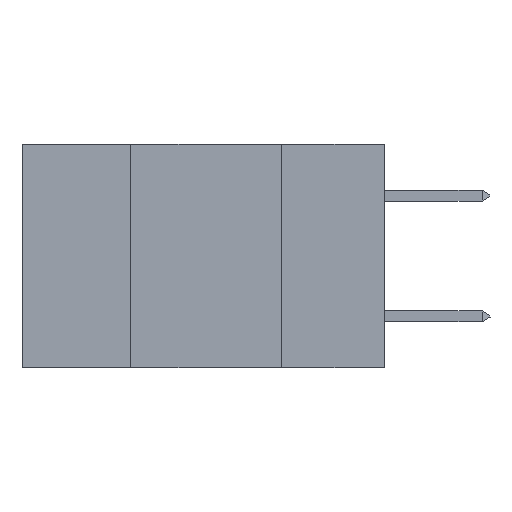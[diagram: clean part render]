
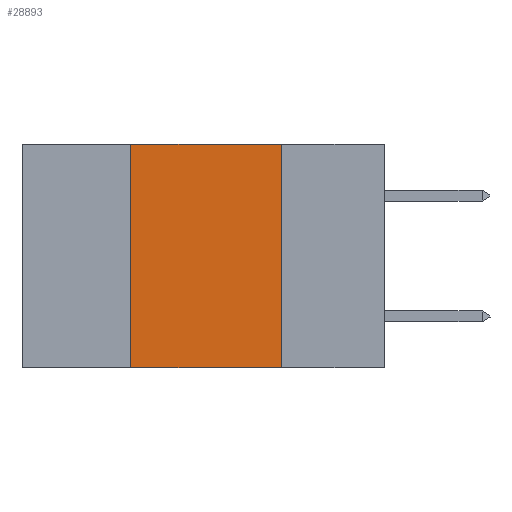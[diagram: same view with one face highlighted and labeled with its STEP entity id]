
A CAD part, left-side view. The second image highlights one B-rep face of the part: STEP entity #28893.
In plain terms, the highlighted planar face has unit normal (-1, 0, 0).
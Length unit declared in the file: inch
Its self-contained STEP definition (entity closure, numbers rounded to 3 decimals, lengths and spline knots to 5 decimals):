
#1052 = CARTESIAN_POINT ( 'NONE',  ( 0., 0.17, -0.37 ) ) ;
#1614 = ORIENTED_EDGE ( 'NONE', *, *, #23762, .F. ) ;
#2181 = FACE_OUTER_BOUND ( 'NONE', #28817, .T. ) ;
#2776 = EDGE_CURVE ( 'NONE', #21338, #18415, #12879, .T. ) ;
#3061 = LINE ( 'NONE', #16066, #25150 ) ;
#3311 = DIRECTION ( 'NONE',  ( 0., -1., 0. ) ) ;
#3324 = DIRECTION ( 'NONE',  ( 0., 0., 1. ) ) ;
#5458 = ORIENTED_EDGE ( 'NONE', *, *, #2776, .T. ) ;
#6096 = VECTOR ( 'NONE', #20080, 39.37008 ) ;
#8983 = CARTESIAN_POINT ( 'NONE',  ( 0., 0.42, -0.37 ) ) ;
#10614 = CARTESIAN_POINT ( 'NONE',  ( 0., 0.6, 0. ) ) ;
#11341 = VERTEX_POINT ( 'NONE', #28186 ) ;
#12218 = ORIENTED_EDGE ( 'NONE', *, *, #23630, .F. ) ;
#12879 = LINE ( 'NONE', #32663, #6096 ) ;
#14375 = CARTESIAN_POINT ( 'NONE',  ( 0., 0.17, 0. ) ) ;
#15922 = CARTESIAN_POINT ( 'NONE',  ( 0., 0.17, 0. ) ) ;
#16066 = CARTESIAN_POINT ( 'NONE',  ( 0., 0.42, 0. ) ) ;
#16925 = DIRECTION ( 'NONE',  ( 1., 0., 0. ) ) ;
#17274 = AXIS2_PLACEMENT_3D ( 'NONE', #32327, #16925, #19282 ) ;
#18415 = VERTEX_POINT ( 'NONE', #1052 ) ;
#19282 = DIRECTION ( 'NONE',  ( 0., 0., -1. ) ) ;
#20080 = DIRECTION ( 'NONE',  ( 0., -1., 0. ) ) ;
#20553 = VERTEX_POINT ( 'NONE', #14375 ) ;
#21338 = VERTEX_POINT ( 'NONE', #8983 ) ;
#21437 = VECTOR ( 'NONE', #28857, 39.37008 ) ;
#22272 = VECTOR ( 'NONE', #3311, 39.37008 ) ;
#22944 = EDGE_CURVE ( 'NONE', #21338, #11341, #3061, .T. ) ;
#23630 = EDGE_CURVE ( 'NONE', #20553, #18415, #27894, .T. ) ;
#23762 = EDGE_CURVE ( 'NONE', #11341, #20553, #25463, .T. ) ;
#24698 = PLANE ( 'NONE',  #17274 ) ;
#25150 = VECTOR ( 'NONE', #3324, 39.37008 ) ;
#25361 = ORIENTED_EDGE ( 'NONE', *, *, #22944, .F. ) ;
#25463 = LINE ( 'NONE', #10614, #22272 ) ;
#27894 = LINE ( 'NONE', #15922, #21437 ) ;
#28186 = CARTESIAN_POINT ( 'NONE',  ( 0., 0.42, 0. ) ) ;
#28817 = EDGE_LOOP ( 'NONE', ( #12218, #1614, #25361, #5458 ) ) ;
#28857 = DIRECTION ( 'NONE',  ( 0., 0., -1. ) ) ;
#28893 = ADVANCED_FACE ( 'NONE', ( #2181 ), #24698, .F. ) ;
#32327 = CARTESIAN_POINT ( 'NONE',  ( 0., 0.6, 0. ) ) ;
#32663 = CARTESIAN_POINT ( 'NONE',  ( 0., 0.6, -0.37 ) ) ;
